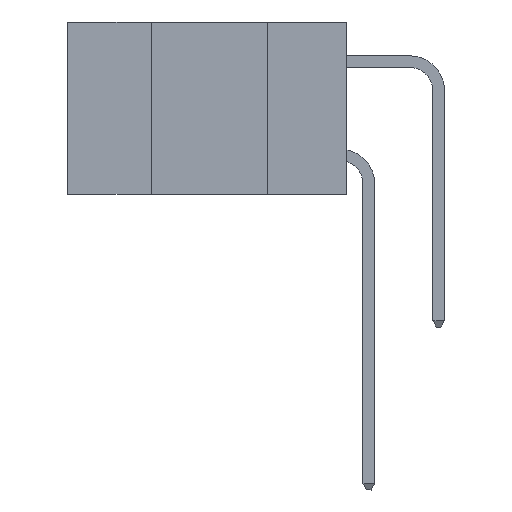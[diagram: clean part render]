
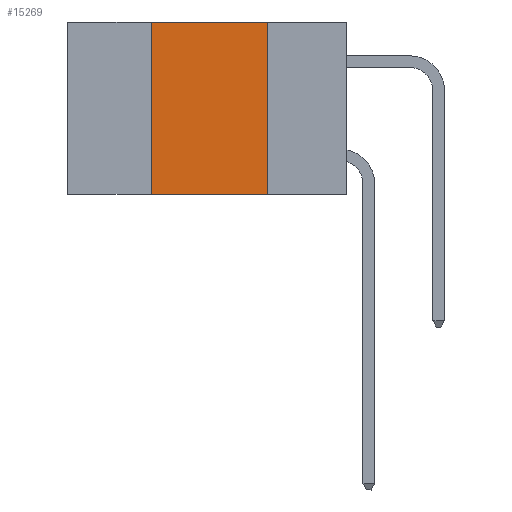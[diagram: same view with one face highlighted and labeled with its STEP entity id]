
A CAD part, left-side view. The second image highlights one B-rep face of the part: STEP entity #15269.
In plain terms, the highlighted planar face has unit normal (-1, 0, 0).
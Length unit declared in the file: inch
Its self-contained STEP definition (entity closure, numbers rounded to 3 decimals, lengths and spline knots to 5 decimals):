
#4 = DIRECTION ( 'NONE',  ( 0., 0., -1. ) ) ;
#752 = DIRECTION ( 'NONE',  ( 0., 0., -1. ) ) ;
#801 = CARTESIAN_POINT ( 'NONE',  ( 0., 0.6, 0. ) ) ;
#1740 = LINE ( 'NONE', #9382, #10344 ) ;
#2250 = CARTESIAN_POINT ( 'NONE',  ( 0., 0.6, -0.37 ) ) ;
#2619 = LINE ( 'NONE', #14064, #4728 ) ;
#2694 = ORIENTED_EDGE ( 'NONE', *, *, #11000, .F. ) ;
#2850 = EDGE_CURVE ( 'NONE', #6898, #5445, #2619, .T. ) ;
#3970 = DIRECTION ( 'NONE',  ( 0., -1., 0. ) ) ;
#4728 = VECTOR ( 'NONE', #4, 39.37008 ) ;
#5061 = VECTOR ( 'NONE', #14622, 39.37008 ) ;
#5226 = VERTEX_POINT ( 'NONE', #11890 ) ;
#5445 = VERTEX_POINT ( 'NONE', #14917 ) ;
#6802 = DIRECTION ( 'NONE',  ( 0., 0., 1. ) ) ;
#6898 = VERTEX_POINT ( 'NONE', #15664 ) ;
#7042 = VERTEX_POINT ( 'NONE', #9634 ) ;
#7052 = EDGE_LOOP ( 'NONE', ( #10524, #2694, #11825, #10729 ) ) ;
#7099 = LINE ( 'NONE', #801, #5061 ) ;
#7781 = AXIS2_PLACEMENT_3D ( 'NONE', #12193, #13266, #752 ) ;
#8304 = VECTOR ( 'NONE', #3970, 39.37008 ) ;
#9382 = CARTESIAN_POINT ( 'NONE',  ( 0., 0.42, 0. ) ) ;
#9634 = CARTESIAN_POINT ( 'NONE',  ( 0., 0.42, -0.37 ) ) ;
#10344 = VECTOR ( 'NONE', #6802, 39.37008 ) ;
#10524 = ORIENTED_EDGE ( 'NONE', *, *, #2850, .F. ) ;
#10729 = ORIENTED_EDGE ( 'NONE', *, *, #15262, .T. ) ;
#11000 = EDGE_CURVE ( 'NONE', #5226, #6898, #7099, .T. ) ;
#11127 = PLANE ( 'NONE',  #7781 ) ;
#11825 = ORIENTED_EDGE ( 'NONE', *, *, #12284, .F. ) ;
#11890 = CARTESIAN_POINT ( 'NONE',  ( 0., 0.42, 0. ) ) ;
#12193 = CARTESIAN_POINT ( 'NONE',  ( 0., 0.6, 0. ) ) ;
#12284 = EDGE_CURVE ( 'NONE', #7042, #5226, #1740, .T. ) ;
#13266 = DIRECTION ( 'NONE',  ( 1., 0., 0. ) ) ;
#13692 = FACE_OUTER_BOUND ( 'NONE', #7052, .T. ) ;
#14064 = CARTESIAN_POINT ( 'NONE',  ( 0., 0.17, 0. ) ) ;
#14622 = DIRECTION ( 'NONE',  ( 0., -1., 0. ) ) ;
#14917 = CARTESIAN_POINT ( 'NONE',  ( 0., 0.17, -0.37 ) ) ;
#15262 = EDGE_CURVE ( 'NONE', #7042, #5445, #15315, .T. ) ;
#15269 = ADVANCED_FACE ( 'NONE', ( #13692 ), #11127, .F. ) ;
#15315 = LINE ( 'NONE', #2250, #8304 ) ;
#15664 = CARTESIAN_POINT ( 'NONE',  ( 0., 0.17, 0. ) ) ;
